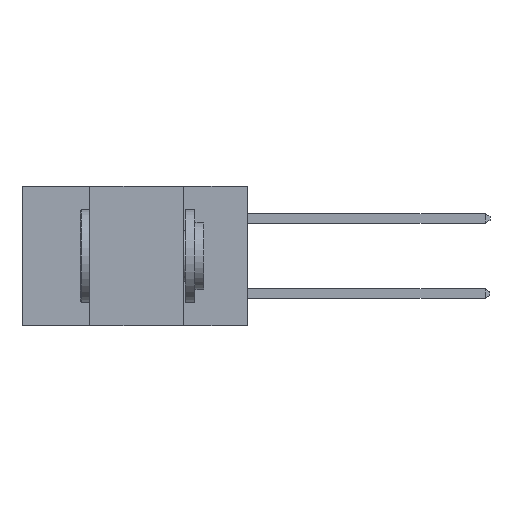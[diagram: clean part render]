
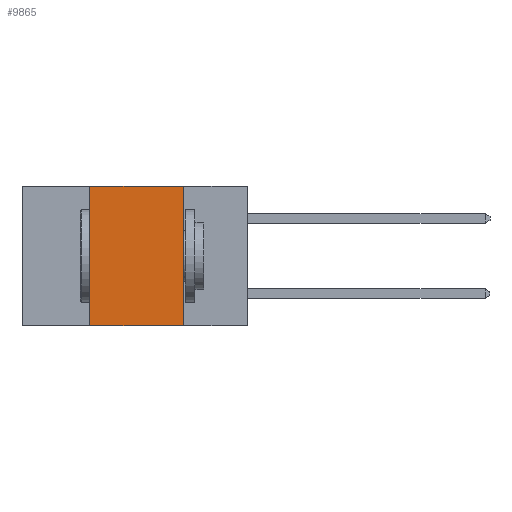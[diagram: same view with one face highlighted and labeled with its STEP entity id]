
A CAD part, left-side view. The second image highlights one B-rep face of the part: STEP entity #9865.
In plain terms, the highlighted planar face has unit normal (-1, 0, 0).
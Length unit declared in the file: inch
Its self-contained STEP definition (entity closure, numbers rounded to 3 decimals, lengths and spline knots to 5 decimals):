
#61 = CARTESIAN_POINT ( 'NONE',  ( 0., 0.42, 0. ) ) ;
#409 = VERTEX_POINT ( 'NONE', #19070 ) ;
#574 = VERTEX_POINT ( 'NONE', #61 ) ;
#985 = PLANE ( 'NONE',  #12663 ) ;
#1570 = CARTESIAN_POINT ( 'NONE',  ( 0., 0.17, 0. ) ) ;
#1629 = CARTESIAN_POINT ( 'NONE',  ( 0., 0.42, 0. ) ) ;
#1683 = LINE ( 'NONE', #1629, #16503 ) ;
#2440 = DIRECTION ( 'NONE',  ( 1., 0., 0. ) ) ;
#3084 = LINE ( 'NONE', #12341, #18388 ) ;
#3262 = EDGE_CURVE ( 'NONE', #409, #16973, #13837, .T. ) ;
#3911 = EDGE_CURVE ( 'NONE', #6997, #16973, #3084, .T. ) ;
#5808 = DIRECTION ( 'NONE',  ( 0., -1., 0. ) ) ;
#5893 = VECTOR ( 'NONE', #9045, 39.37008 ) ;
#5982 = EDGE_LOOP ( 'NONE', ( #15710, #13677, #9842, #18839 ) ) ;
#6395 = EDGE_CURVE ( 'NONE', #574, #409, #13966, .T. ) ;
#6997 = VERTEX_POINT ( 'NONE', #18876 ) ;
#9045 = DIRECTION ( 'NONE',  ( 0., 0., -1. ) ) ;
#9842 = ORIENTED_EDGE ( 'NONE', *, *, #17967, .F. ) ;
#9865 = ADVANCED_FACE ( 'NONE', ( #10017 ), #985, .F. ) ;
#9998 = VECTOR ( 'NONE', #5808, 39.37008 ) ;
#10002 = CARTESIAN_POINT ( 'NONE',  ( 0., 0.17, -0.37 ) ) ;
#10017 = FACE_OUTER_BOUND ( 'NONE', #5982, .T. ) ;
#11290 = CARTESIAN_POINT ( 'NONE',  ( 0., 0.6, 0. ) ) ;
#11876 = CARTESIAN_POINT ( 'NONE',  ( 0., 0.6, 0. ) ) ;
#12341 = CARTESIAN_POINT ( 'NONE',  ( 0., 0.6, -0.37 ) ) ;
#12631 = DIRECTION ( 'NONE',  ( 0., -1., 0. ) ) ;
#12663 = AXIS2_PLACEMENT_3D ( 'NONE', #11290, #2440, #12840 ) ;
#12840 = DIRECTION ( 'NONE',  ( 0., 0., -1. ) ) ;
#13677 = ORIENTED_EDGE ( 'NONE', *, *, #6395, .F. ) ;
#13837 = LINE ( 'NONE', #1570, #5893 ) ;
#13966 = LINE ( 'NONE', #11876, #9998 ) ;
#15710 = ORIENTED_EDGE ( 'NONE', *, *, #3262, .F. ) ;
#16503 = VECTOR ( 'NONE', #17938, 39.37008 ) ;
#16973 = VERTEX_POINT ( 'NONE', #10002 ) ;
#17938 = DIRECTION ( 'NONE',  ( 0., 0., 1. ) ) ;
#17967 = EDGE_CURVE ( 'NONE', #6997, #574, #1683, .T. ) ;
#18388 = VECTOR ( 'NONE', #12631, 39.37008 ) ;
#18839 = ORIENTED_EDGE ( 'NONE', *, *, #3911, .T. ) ;
#18876 = CARTESIAN_POINT ( 'NONE',  ( 0., 0.42, -0.37 ) ) ;
#19070 = CARTESIAN_POINT ( 'NONE',  ( 0., 0.17, 0. ) ) ;
